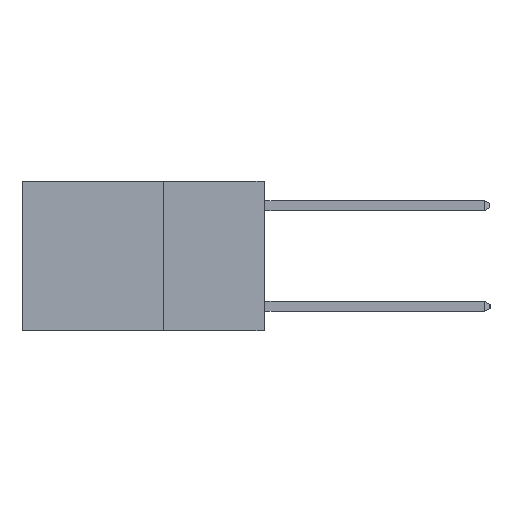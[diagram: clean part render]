
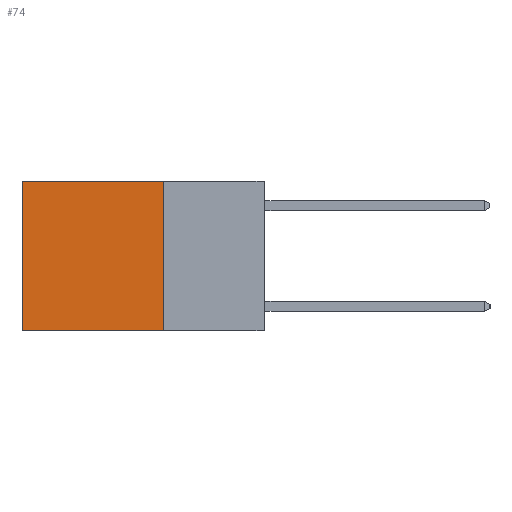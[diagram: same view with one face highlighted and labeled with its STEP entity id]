
A CAD part, left-side view. The second image highlights one B-rep face of the part: STEP entity #74.
In plain terms, the highlighted planar face has unit normal (-1, 0, 0).
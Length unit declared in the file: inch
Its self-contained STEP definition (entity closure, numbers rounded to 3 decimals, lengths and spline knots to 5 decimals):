
#26 = CARTESIAN_POINT ( 'NONE',  ( 0.2625, 0.25, 0. ) ) ;
#56 = PLANE ( 'NONE',  #3897 ) ;
#74 = ADVANCED_FACE ( 'NONE', ( #7663 ), #56, .F. ) ;
#1124 = DIRECTION ( 'NONE',  ( 0., 0., -1. ) ) ;
#1198 = LINE ( 'NONE', #26, #5247 ) ;
#1519 = CARTESIAN_POINT ( 'NONE',  ( 0.2625, 0.25, -0.37 ) ) ;
#1787 = EDGE_CURVE ( 'NONE', #5744, #8553, #4342, .T. ) ;
#1832 = CARTESIAN_POINT ( 'NONE',  ( 0.2625, 0.6, 0. ) ) ;
#1926 = DIRECTION ( 'NONE',  ( 0., 1., 0. ) ) ;
#2061 = CARTESIAN_POINT ( 'NONE',  ( 0.2625, 0.25, 0. ) ) ;
#2230 = VECTOR ( 'NONE', #1124, 39.37008 ) ;
#2366 = ORIENTED_EDGE ( 'NONE', *, *, #9071, .T. ) ;
#2368 = EDGE_CURVE ( 'NONE', #9417, #6258, #9720, .T. ) ;
#2706 = DIRECTION ( 'NONE',  ( 0., 1., 0. ) ) ;
#2767 = VECTOR ( 'NONE', #1926, 39.37008 ) ;
#2884 = DIRECTION ( 'NONE',  ( 0., 0., -1. ) ) ;
#3411 = DIRECTION ( 'NONE',  ( 0., 0., -1. ) ) ;
#3897 = AXIS2_PLACEMENT_3D ( 'NONE', #5498, #8939, #3411 ) ;
#3973 = ORIENTED_EDGE ( 'NONE', *, *, #1787, .T. ) ;
#4342 = LINE ( 'NONE', #9143, #2230 ) ;
#5247 = VECTOR ( 'NONE', #2706, 39.37008 ) ;
#5413 = EDGE_LOOP ( 'NONE', ( #3973, #6308, #8419, #2366 ) ) ;
#5498 = CARTESIAN_POINT ( 'NONE',  ( 0.2625, 0.25, 0. ) ) ;
#5744 = VERTEX_POINT ( 'NONE', #1832 ) ;
#6258 = VERTEX_POINT ( 'NONE', #1519 ) ;
#6308 = ORIENTED_EDGE ( 'NONE', *, *, #9863, .F. ) ;
#7564 = CARTESIAN_POINT ( 'NONE',  ( 0.2625, 0.6, -0.37 ) ) ;
#7569 = VECTOR ( 'NONE', #2884, 39.37008 ) ;
#7663 = FACE_OUTER_BOUND ( 'NONE', #5413, .T. ) ;
#8235 = CARTESIAN_POINT ( 'NONE',  ( 0.2625, 0.25, -0.37 ) ) ;
#8419 = ORIENTED_EDGE ( 'NONE', *, *, #2368, .F. ) ;
#8553 = VERTEX_POINT ( 'NONE', #7564 ) ;
#8939 = DIRECTION ( 'NONE',  ( 1., 0., 0. ) ) ;
#9071 = EDGE_CURVE ( 'NONE', #9417, #5744, #1198, .T. ) ;
#9098 = LINE ( 'NONE', #8235, #2767 ) ;
#9143 = CARTESIAN_POINT ( 'NONE',  ( 0.2625, 0.6, 0. ) ) ;
#9417 = VERTEX_POINT ( 'NONE', #10210 ) ;
#9720 = LINE ( 'NONE', #2061, #7569 ) ;
#9863 = EDGE_CURVE ( 'NONE', #6258, #8553, #9098, .T. ) ;
#10210 = CARTESIAN_POINT ( 'NONE',  ( 0.2625, 0.25, 0. ) ) ;
